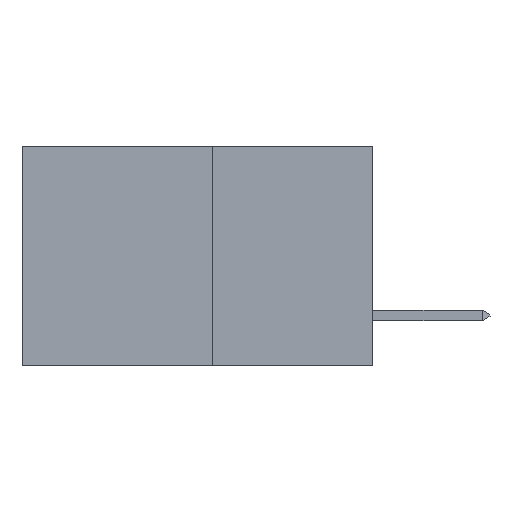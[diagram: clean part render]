
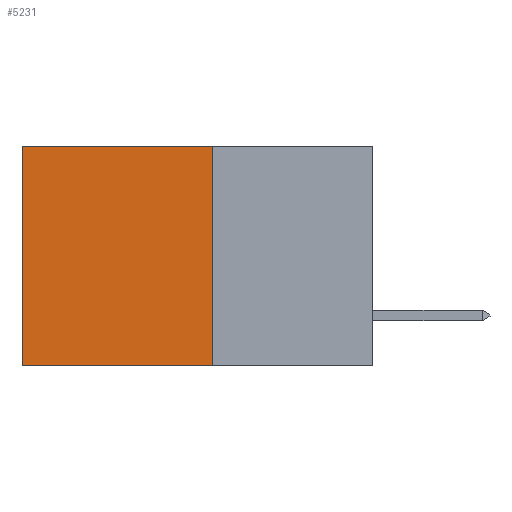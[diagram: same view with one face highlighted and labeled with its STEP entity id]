
A CAD part, left-side view. The second image highlights one B-rep face of the part: STEP entity #5231.
In plain terms, the highlighted planar face has unit normal (-1, 0, 0).
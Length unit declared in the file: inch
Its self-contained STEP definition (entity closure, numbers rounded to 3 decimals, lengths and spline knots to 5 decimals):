
#156 = VECTOR ( 'NONE', #5674, 39.37008 ) ;
#362 = LINE ( 'NONE', #5080, #10364 ) ;
#442 = DIRECTION ( 'NONE',  ( 0., 0., -1. ) ) ;
#482 = DIRECTION ( 'NONE',  ( 1., 0., 0. ) ) ;
#522 = LINE ( 'NONE', #9672, #10237 ) ;
#576 = VERTEX_POINT ( 'NONE', #3417 ) ;
#722 = CARTESIAN_POINT ( 'NONE',  ( 0.277, 0.27, -0.37 ) ) ;
#853 = PLANE ( 'NONE',  #10791 ) ;
#916 = ORIENTED_EDGE ( 'NONE', *, *, #1376, .F. ) ;
#956 = ORIENTED_EDGE ( 'NONE', *, *, #7284, .T. ) ;
#1240 = ORIENTED_EDGE ( 'NONE', *, *, #1704, .F. ) ;
#1376 = EDGE_CURVE ( 'NONE', #6367, #11465, #2999, .T. ) ;
#1436 = CARTESIAN_POINT ( 'NONE',  ( 0.277, 0.27, -0.37 ) ) ;
#1553 = CARTESIAN_POINT ( 'NONE',  ( 0.277, 0.59, -0.37 ) ) ;
#1704 = EDGE_CURVE ( 'NONE', #11465, #6496, #8568, .T. ) ;
#2182 = DIRECTION ( 'NONE',  ( 0., 0., -1. ) ) ;
#2391 = EDGE_LOOP ( 'NONE', ( #3944, #1240, #916, #956 ) ) ;
#2999 = LINE ( 'NONE', #11619, #156 ) ;
#3417 = CARTESIAN_POINT ( 'NONE',  ( 0.277, 0.59, 0. ) ) ;
#3944 = ORIENTED_EDGE ( 'NONE', *, *, #11545, .T. ) ;
#4880 = CARTESIAN_POINT ( 'NONE',  ( 0.277, 0.27, -0.37 ) ) ;
#5080 = CARTESIAN_POINT ( 'NONE',  ( 0.277, 0.27, 0. ) ) ;
#5091 = DIRECTION ( 'NONE',  ( 0., 1., 0. ) ) ;
#5231 = ADVANCED_FACE ( 'NONE', ( #11428 ), #853, .F. ) ;
#5322 = CARTESIAN_POINT ( 'NONE',  ( 0.277, 0.27, 0. ) ) ;
#5674 = DIRECTION ( 'NONE',  ( 0., 0., -1. ) ) ;
#6343 = VECTOR ( 'NONE', #9096, 39.37008 ) ;
#6367 = VERTEX_POINT ( 'NONE', #5322 ) ;
#6496 = VERTEX_POINT ( 'NONE', #1553 ) ;
#7284 = EDGE_CURVE ( 'NONE', #6367, #576, #362, .T. ) ;
#8568 = LINE ( 'NONE', #1436, #6343 ) ;
#9096 = DIRECTION ( 'NONE',  ( 0., 1., 0. ) ) ;
#9672 = CARTESIAN_POINT ( 'NONE',  ( 0.277, 0.59, -0.37 ) ) ;
#10237 = VECTOR ( 'NONE', #2182, 39.37008 ) ;
#10364 = VECTOR ( 'NONE', #5091, 39.37008 ) ;
#10791 = AXIS2_PLACEMENT_3D ( 'NONE', #722, #482, #442 ) ;
#11428 = FACE_OUTER_BOUND ( 'NONE', #2391, .T. ) ;
#11465 = VERTEX_POINT ( 'NONE', #4880 ) ;
#11545 = EDGE_CURVE ( 'NONE', #576, #6496, #522, .T. ) ;
#11619 = CARTESIAN_POINT ( 'NONE',  ( 0.277, 0.27, -0.37 ) ) ;
